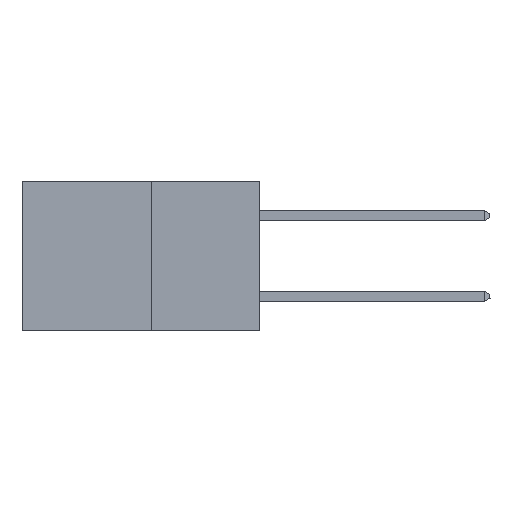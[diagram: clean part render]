
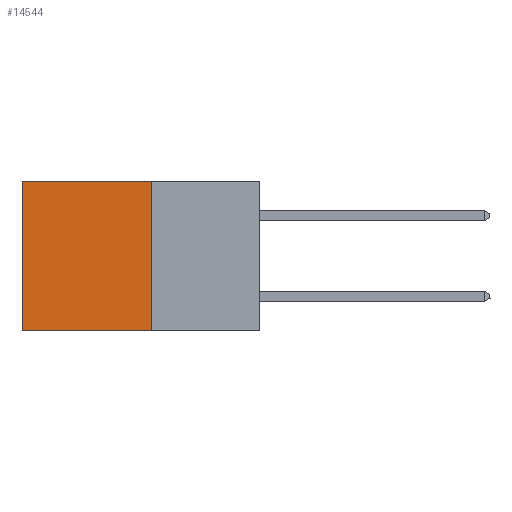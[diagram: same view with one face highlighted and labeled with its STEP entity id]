
A CAD part, left-side view. The second image highlights one B-rep face of the part: STEP entity #14544.
In plain terms, the highlighted planar face has unit normal (-1, 0, 0).
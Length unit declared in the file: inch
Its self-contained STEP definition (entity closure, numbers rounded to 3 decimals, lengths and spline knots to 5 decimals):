
#23 = DIRECTION ( 'NONE',  ( 1., 0., 0. ) ) ;
#189 = ORIENTED_EDGE ( 'NONE', *, *, #5651, .T. ) ;
#343 = FACE_OUTER_BOUND ( 'NONE', #12619, .T. ) ;
#735 = VERTEX_POINT ( 'NONE', #17642 ) ;
#2353 = CARTESIAN_POINT ( 'NONE',  ( 0.277, 0.27, -0.37 ) ) ;
#2708 = DIRECTION ( 'NONE',  ( 0., 1., 0. ) ) ;
#2979 = CARTESIAN_POINT ( 'NONE',  ( 0.277, 0.27, -0.37 ) ) ;
#3391 = VERTEX_POINT ( 'NONE', #4776 ) ;
#4776 = CARTESIAN_POINT ( 'NONE',  ( 0.277, 0.59, -0.37 ) ) ;
#4999 = VECTOR ( 'NONE', #15278, 39.37008 ) ;
#5332 = PLANE ( 'NONE',  #8427 ) ;
#5651 = EDGE_CURVE ( 'NONE', #735, #11652, #8902, .T. ) ;
#6917 = EDGE_CURVE ( 'NONE', #11652, #3391, #7160, .T. ) ;
#6956 = CARTESIAN_POINT ( 'NONE',  ( 0.277, 0.27, -0.37 ) ) ;
#7160 = LINE ( 'NONE', #11754, #14127 ) ;
#7329 = VECTOR ( 'NONE', #2708, 39.37008 ) ;
#8015 = EDGE_CURVE ( 'NONE', #12231, #3391, #11019, .T. ) ;
#8427 = AXIS2_PLACEMENT_3D ( 'NONE', #14996, #23, #9485 ) ;
#8902 = LINE ( 'NONE', #14279, #15874 ) ;
#9017 = ORIENTED_EDGE ( 'NONE', *, *, #8015, .F. ) ;
#9485 = DIRECTION ( 'NONE',  ( 0., 0., -1. ) ) ;
#10180 = CARTESIAN_POINT ( 'NONE',  ( 0.277, 0.59, 0. ) ) ;
#11019 = LINE ( 'NONE', #2979, #7329 ) ;
#11117 = ORIENTED_EDGE ( 'NONE', *, *, #6917, .T. ) ;
#11652 = VERTEX_POINT ( 'NONE', #10180 ) ;
#11733 = DIRECTION ( 'NONE',  ( 0., 0., -1. ) ) ;
#11754 = CARTESIAN_POINT ( 'NONE',  ( 0.277, 0.59, -0.37 ) ) ;
#12231 = VERTEX_POINT ( 'NONE', #2353 ) ;
#12619 = EDGE_LOOP ( 'NONE', ( #11117, #9017, #15741, #189 ) ) ;
#12731 = LINE ( 'NONE', #6956, #4999 ) ;
#13260 = EDGE_CURVE ( 'NONE', #735, #12231, #12731, .T. ) ;
#14094 = DIRECTION ( 'NONE',  ( 0., 1., 0. ) ) ;
#14127 = VECTOR ( 'NONE', #11733, 39.37008 ) ;
#14279 = CARTESIAN_POINT ( 'NONE',  ( 0.277, 0.27, 0. ) ) ;
#14544 = ADVANCED_FACE ( 'NONE', ( #343 ), #5332, .F. ) ;
#14996 = CARTESIAN_POINT ( 'NONE',  ( 0.277, 0.27, -0.37 ) ) ;
#15278 = DIRECTION ( 'NONE',  ( 0., 0., -1. ) ) ;
#15741 = ORIENTED_EDGE ( 'NONE', *, *, #13260, .F. ) ;
#15874 = VECTOR ( 'NONE', #14094, 39.37008 ) ;
#17642 = CARTESIAN_POINT ( 'NONE',  ( 0.277, 0.27, 0. ) ) ;
